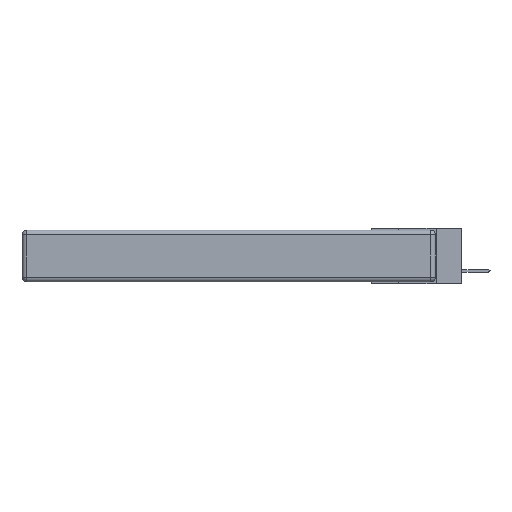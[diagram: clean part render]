
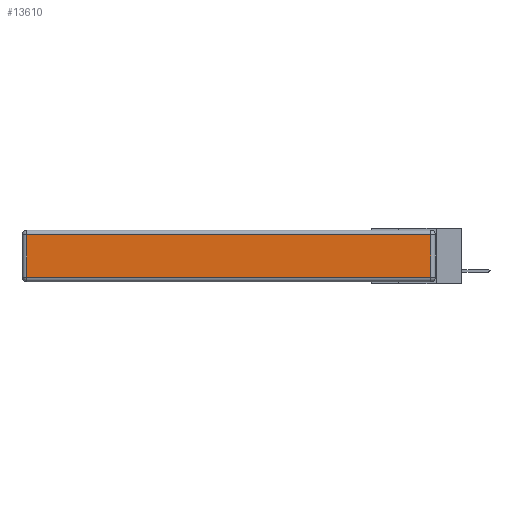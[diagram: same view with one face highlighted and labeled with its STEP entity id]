
A CAD part, left-side view. The second image highlights one B-rep face of the part: STEP entity #13610.
In plain terms, the highlighted planar face has unit normal (-1, 0, 0).
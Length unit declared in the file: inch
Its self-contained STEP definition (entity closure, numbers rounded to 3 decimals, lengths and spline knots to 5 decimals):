
#376 = VECTOR ( 'NONE', #10066, 39.37008 ) ;
#1262 = LINE ( 'NONE', #3569, #2089 ) ;
#1551 = VERTEX_POINT ( 'NONE', #13030 ) ;
#2089 = VECTOR ( 'NONE', #3426, 39.37008 ) ;
#2222 = ORIENTED_EDGE ( 'NONE', *, *, #2920, .T. ) ;
#2316 = VERTEX_POINT ( 'NONE', #5543 ) ;
#2419 = VERTEX_POINT ( 'NONE', #9373 ) ;
#2594 = CARTESIAN_POINT ( 'NONE',  ( 0., 0., -0.313 ) ) ;
#2621 = DIRECTION ( 'NONE',  ( -1., 0., 0. ) ) ;
#2920 = EDGE_CURVE ( 'NONE', #2316, #2419, #1262, .T. ) ;
#2964 = ORIENTED_EDGE ( 'NONE', *, *, #9518, .T. ) ;
#3233 = PLANE ( 'NONE',  #8291 ) ;
#3327 = EDGE_CURVE ( 'NONE', #2419, #1551, #13038, .T. ) ;
#3426 = DIRECTION ( 'NONE',  ( 0., 1., 0. ) ) ;
#3569 = CARTESIAN_POINT ( 'NONE',  ( 0., 2.75, -0.03 ) ) ;
#4631 = DIRECTION ( 'NONE',  ( 0., 0., 1. ) ) ;
#5035 = VECTOR ( 'NONE', #13023, 39.37008 ) ;
#5253 = FACE_OUTER_BOUND ( 'NONE', #11019, .T. ) ;
#5487 = CARTESIAN_POINT ( 'NONE',  ( 0., 0.03, -0.313 ) ) ;
#5543 = CARTESIAN_POINT ( 'NONE',  ( 0., 0.03, -0.03 ) ) ;
#6748 = ORIENTED_EDGE ( 'NONE', *, *, #12674, .T. ) ;
#7014 = CARTESIAN_POINT ( 'NONE',  ( 0., 0., -0.343 ) ) ;
#7118 = VERTEX_POINT ( 'NONE', #5487 ) ;
#7868 = DIRECTION ( 'NONE',  ( 0., -1., 0. ) ) ;
#7911 = LINE ( 'NONE', #9659, #5035 ) ;
#8291 = AXIS2_PLACEMENT_3D ( 'NONE', #7014, #2621, #4631 ) ;
#8471 = LINE ( 'NONE', #2594, #8644 ) ;
#8644 = VECTOR ( 'NONE', #7868, 39.37008 ) ;
#8984 = CARTESIAN_POINT ( 'NONE',  ( 0., 2.72, -0.343 ) ) ;
#9373 = CARTESIAN_POINT ( 'NONE',  ( 0., 2.72, -0.03 ) ) ;
#9518 = EDGE_CURVE ( 'NONE', #7118, #2316, #7911, .T. ) ;
#9659 = CARTESIAN_POINT ( 'NONE',  ( 0., 0.03, -0.343 ) ) ;
#10066 = DIRECTION ( 'NONE',  ( 0., 0., -1. ) ) ;
#10857 = ORIENTED_EDGE ( 'NONE', *, *, #3327, .T. ) ;
#11019 = EDGE_LOOP ( 'NONE', ( #6748, #2964, #2222, #10857 ) ) ;
#12674 = EDGE_CURVE ( 'NONE', #1551, #7118, #8471, .T. ) ;
#13023 = DIRECTION ( 'NONE',  ( 0., 0., 1. ) ) ;
#13030 = CARTESIAN_POINT ( 'NONE',  ( 0., 2.72, -0.313 ) ) ;
#13038 = LINE ( 'NONE', #8984, #376 ) ;
#13610 = ADVANCED_FACE ( 'NONE', ( #5253 ), #3233, .T. ) ;
